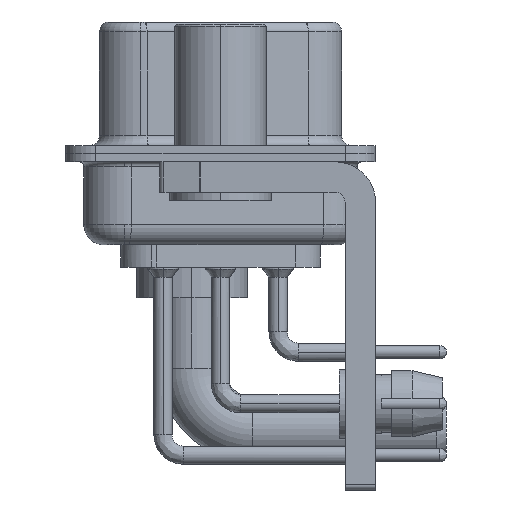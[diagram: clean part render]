
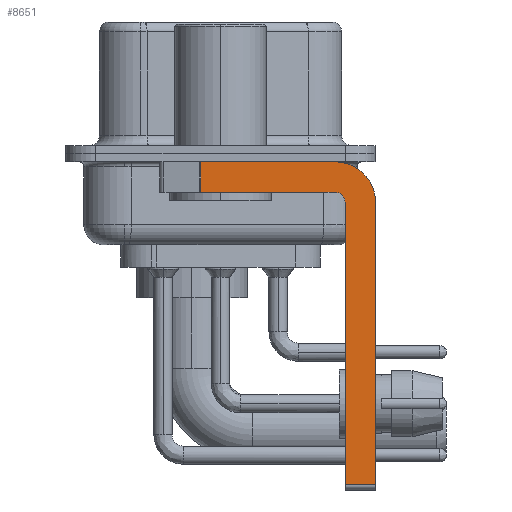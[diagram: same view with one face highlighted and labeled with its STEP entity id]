
A CAD part, left-side view. The second image highlights one B-rep face of the part: STEP entity #8651.
In plain terms, the highlighted planar face has unit normal (-1, 0, 0).
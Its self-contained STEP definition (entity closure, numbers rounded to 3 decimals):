
#9 = AXIS2_PLACEMENT_3D ( 'NONE', #22013, #26001, #16130 ) ;
#2080 = LINE ( 'NONE', #27737, #37355 ) ;
#3234 = DIRECTION ( 'NONE',  ( 0., 0., -1. ) ) ;
#3994 = ORIENTED_EDGE ( 'NONE', *, *, #26358, .T. ) ;
#3997 = EDGE_CURVE ( 'NONE', #15216, #20002, #19333, .T. ) ;
#4447 = DIRECTION ( 'NONE',  ( 0., 1., 0. ) ) ;
#7432 = AXIS2_PLACEMENT_3D ( 'NONE', #9876, #22681, #35519 ) ;
#8342 = VERTEX_POINT ( 'NONE', #14537 ) ;
#8651 = ADVANCED_FACE ( 'NONE', ( #28589 ), #25845, .F. ) ;
#8803 = ORIENTED_EDGE ( 'NONE', *, *, #19457, .F. ) ;
#9134 = EDGE_CURVE ( 'NONE', #20002, #24144, #25517, .T. ) ;
#9462 = CARTESIAN_POINT ( 'NONE',  ( -2.9, 3., -0.4 ) ) ;
#9876 = CARTESIAN_POINT ( 'NONE',  ( -2.9, -5.65, -2.4 ) ) ;
#10562 = ORIENTED_EDGE ( 'NONE', *, *, #15122, .F. ) ;
#10951 = ORIENTED_EDGE ( 'NONE', *, *, #21571, .T. ) ;
#11455 = LINE ( 'NONE', #21519, #41036 ) ;
#12088 = CARTESIAN_POINT ( 'NONE',  ( -2.9, -5.65, -2.4 ) ) ;
#12278 = CARTESIAN_POINT ( 'NONE',  ( -2.9, -7.65, -2.4 ) ) ;
#12901 = CARTESIAN_POINT ( 'NONE',  ( -2.9, 0.978, -0.4 ) ) ;
#13382 = EDGE_LOOP ( 'NONE', ( #32011, #3994, #8803, #10562, #20904, #10951, #14719, #39918 ) ) ;
#14537 = CARTESIAN_POINT ( 'NONE',  ( -2.9, -6.15, -16.35 ) ) ;
#14719 = ORIENTED_EDGE ( 'NONE', *, *, #33877, .F. ) ;
#15122 = EDGE_CURVE ( 'NONE', #24864, #28276, #17779, .T. ) ;
#15216 = VERTEX_POINT ( 'NONE', #12901 ) ;
#16130 = DIRECTION ( 'NONE',  ( 0., 0., -1. ) ) ;
#17779 = CIRCLE ( 'NONE', #41271, 0.5 ) ;
#18392 = VECTOR ( 'NONE', #38870, 1000. ) ;
#18674 = LINE ( 'NONE', #21816, #24087 ) ;
#19333 = LINE ( 'NONE', #9462, #18392 ) ;
#19457 = EDGE_CURVE ( 'NONE', #28276, #32900, #39327, .T. ) ;
#20002 = VERTEX_POINT ( 'NONE', #20558 ) ;
#20558 = CARTESIAN_POINT ( 'NONE',  ( -2.9, -5.65, -0.4 ) ) ;
#20904 = ORIENTED_EDGE ( 'NONE', *, *, #33776, .F. ) ;
#21175 = CARTESIAN_POINT ( 'NONE',  ( -2.9, -5.65, -1.9 ) ) ;
#21519 = CARTESIAN_POINT ( 'NONE',  ( -2.9, -6.15, -16.6 ) ) ;
#21571 = EDGE_CURVE ( 'NONE', #8342, #27913, #18674, .T. ) ;
#21816 = CARTESIAN_POINT ( 'NONE',  ( -2.9, -5.65, -16.35 ) ) ;
#22013 = CARTESIAN_POINT ( 'NONE',  ( -2.9, -5.65, -2.4 ) ) ;
#22681 = DIRECTION ( 'NONE',  ( 1., 0., 0. ) ) ;
#23354 = CARTESIAN_POINT ( 'NONE',  ( -2.9, -5.65, -1.9 ) ) ;
#24087 = VECTOR ( 'NONE', #31502, 1000. ) ;
#24144 = VERTEX_POINT ( 'NONE', #12278 ) ;
#24864 = VERTEX_POINT ( 'NONE', #29842 ) ;
#25096 = DIRECTION ( 'NONE',  ( 0., 0., 1. ) ) ;
#25517 = CIRCLE ( 'NONE', #9, 2. ) ;
#25845 = PLANE ( 'NONE',  #7432 ) ;
#26001 = DIRECTION ( 'NONE',  ( 1., 0., 0. ) ) ;
#26358 = EDGE_CURVE ( 'NONE', #15216, #32900, #2080, .T. ) ;
#27633 = DIRECTION ( 'NONE',  ( 0., 0., 1. ) ) ;
#27737 = CARTESIAN_POINT ( 'NONE',  ( -2.9, 0.978, -1.9 ) ) ;
#27913 = VERTEX_POINT ( 'NONE', #38654 ) ;
#28276 = VERTEX_POINT ( 'NONE', #21175 ) ;
#28589 = FACE_OUTER_BOUND ( 'NONE', #13382, .T. ) ;
#29842 = CARTESIAN_POINT ( 'NONE',  ( -2.9, -6.15, -2.4 ) ) ;
#30079 = VECTOR ( 'NONE', #4447, 1000. ) ;
#31320 = DIRECTION ( 'NONE',  ( 0., 0., -1. ) ) ;
#31502 = DIRECTION ( 'NONE',  ( 0., -1., 0. ) ) ;
#32011 = ORIENTED_EDGE ( 'NONE', *, *, #3997, .F. ) ;
#32030 = LINE ( 'NONE', #37928, #32967 ) ;
#32900 = VERTEX_POINT ( 'NONE', #34454 ) ;
#32967 = VECTOR ( 'NONE', #3234, 1000. ) ;
#33776 = EDGE_CURVE ( 'NONE', #8342, #24864, #11455, .T. ) ;
#33877 = EDGE_CURVE ( 'NONE', #24144, #27913, #32030, .T. ) ;
#34454 = CARTESIAN_POINT ( 'NONE',  ( -2.9, 0.978, -1.9 ) ) ;
#35519 = DIRECTION ( 'NONE',  ( 0., 0., -1. ) ) ;
#37301 = DIRECTION ( 'NONE',  ( -1., 0., 0. ) ) ;
#37355 = VECTOR ( 'NONE', #31320, 1000. ) ;
#37928 = CARTESIAN_POINT ( 'NONE',  ( -2.9, -7.65, -2.4 ) ) ;
#38654 = CARTESIAN_POINT ( 'NONE',  ( -2.9, -7.65, -16.35 ) ) ;
#38870 = DIRECTION ( 'NONE',  ( 0., -1., 0. ) ) ;
#39327 = LINE ( 'NONE', #23354, #30079 ) ;
#39918 = ORIENTED_EDGE ( 'NONE', *, *, #9134, .F. ) ;
#41036 = VECTOR ( 'NONE', #27633, 1000. ) ;
#41271 = AXIS2_PLACEMENT_3D ( 'NONE', #12088, #37301, #25096 ) ;
